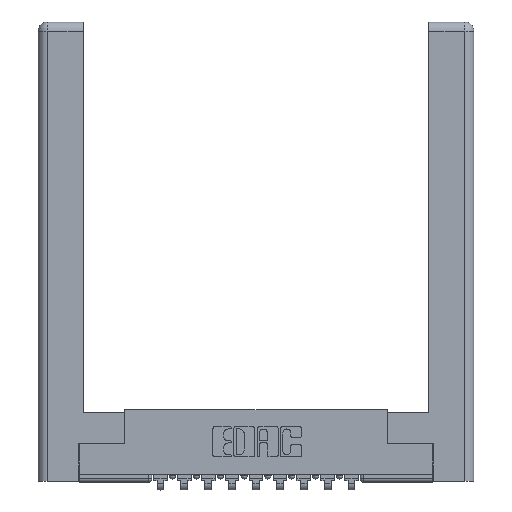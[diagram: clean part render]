
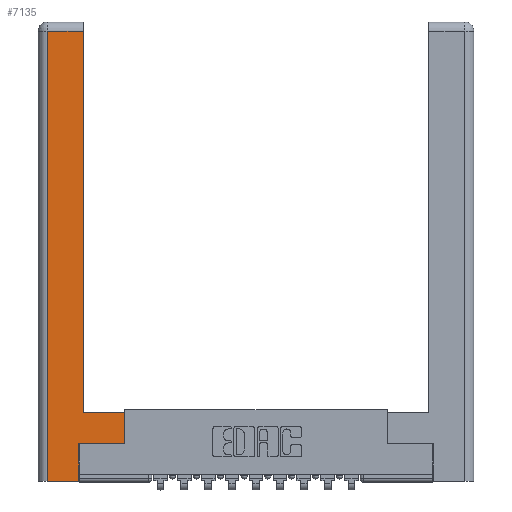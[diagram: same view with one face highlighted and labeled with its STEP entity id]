
A CAD part, top view. The second image highlights one B-rep face of the part: STEP entity #7135.
In plain terms, the highlighted planar face has unit normal (0, 0, 1).
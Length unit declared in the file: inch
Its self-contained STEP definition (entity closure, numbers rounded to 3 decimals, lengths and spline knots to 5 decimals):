
#481 = VECTOR ( 'NONE', #7855, 39.37008 ) ;
#577 = LINE ( 'NONE', #14822, #9826 ) ;
#635 = ORIENTED_EDGE ( 'NONE', *, *, #12212, .T. ) ;
#964 = VERTEX_POINT ( 'NONE', #5883 ) ;
#1213 = CARTESIAN_POINT ( 'NONE',  ( 0.0615, 2.94, 0. ) ) ;
#1228 = LINE ( 'NONE', #13345, #13043 ) ;
#1716 = FACE_OUTER_BOUND ( 'NONE', #7790, .T. ) ;
#1934 = ORIENTED_EDGE ( 'NONE', *, *, #13706, .T. ) ;
#2009 = CARTESIAN_POINT ( 'NONE',  ( 0.565, 0.245, 0. ) ) ;
#2551 = VERTEX_POINT ( 'NONE', #6103 ) ;
#3021 = PLANE ( 'NONE',  #4037 ) ;
#3238 = CARTESIAN_POINT ( 'NONE',  ( 0.565, 0.245, 0. ) ) ;
#3456 = ORIENTED_EDGE ( 'NONE', *, *, #12498, .T. ) ;
#4037 = AXIS2_PLACEMENT_3D ( 'NONE', #10258, #6478, #4224 ) ;
#4224 = DIRECTION ( 'NONE',  ( -1., 0., 0. ) ) ;
#4904 = CARTESIAN_POINT ( 'NONE',  ( 0.265, 0.245, 0. ) ) ;
#4952 = VECTOR ( 'NONE', #8055, 39.37008 ) ;
#5247 = EDGE_CURVE ( 'NONE', #8788, #11403, #8858, .T. ) ;
#5883 = CARTESIAN_POINT ( 'NONE',  ( 0.295, 0.45, 0. ) ) ;
#6103 = CARTESIAN_POINT ( 'NONE',  ( 0.265, 0., 0. ) ) ;
#6108 = ORIENTED_EDGE ( 'NONE', *, *, #14114, .T. ) ;
#6281 = DIRECTION ( 'NONE',  ( 1., 0., 0. ) ) ;
#6478 = DIRECTION ( 'NONE',  ( 0., 0., -1. ) ) ;
#6773 = LINE ( 'NONE', #9092, #481 ) ;
#6838 = ORIENTED_EDGE ( 'NONE', *, *, #13194, .T. ) ;
#6981 = LINE ( 'NONE', #10394, #9014 ) ;
#7135 = ADVANCED_FACE ( 'NONE', ( #1716 ), #3021, .F. ) ;
#7223 = DIRECTION ( 'NONE',  ( 0., 1., 0. ) ) ;
#7790 = EDGE_LOOP ( 'NONE', ( #6108, #635, #9020, #1934, #3456, #8652, #6838, #11118 ) ) ;
#7855 = DIRECTION ( 'NONE',  ( -1., 0., 0. ) ) ;
#8055 = DIRECTION ( 'NONE',  ( 1., 0., 0. ) ) ;
#8219 = LINE ( 'NONE', #13305, #9128 ) ;
#8366 = DIRECTION ( 'NONE',  ( 0., 1., 0. ) ) ;
#8652 = ORIENTED_EDGE ( 'NONE', *, *, #13442, .T. ) ;
#8788 = VERTEX_POINT ( 'NONE', #1213 ) ;
#8858 = LINE ( 'NONE', #14935, #10699 ) ;
#8957 = EDGE_CURVE ( 'NONE', #12801, #964, #577, .T. ) ;
#9014 = VECTOR ( 'NONE', #11666, 39.37008 ) ;
#9020 = ORIENTED_EDGE ( 'NONE', *, *, #5247, .T. ) ;
#9092 = CARTESIAN_POINT ( 'NONE',  ( 0.0615, 2.94, 0. ) ) ;
#9128 = VECTOR ( 'NONE', #8366, 39.37008 ) ;
#9530 = VECTOR ( 'NONE', #7223, 39.37008 ) ;
#9826 = VECTOR ( 'NONE', #12447, 39.37008 ) ;
#10258 = CARTESIAN_POINT ( 'NONE',  ( 0., 0., 0. ) ) ;
#10265 = DIRECTION ( 'NONE',  ( 0., -1., 0. ) ) ;
#10394 = CARTESIAN_POINT ( 'NONE',  ( 0.295, 3., 0. ) ) ;
#10699 = VECTOR ( 'NONE', #10265, 39.37008 ) ;
#10854 = LINE ( 'NONE', #3238, #4952 ) ;
#11009 = LINE ( 'NONE', #4904, #9530 ) ;
#11094 = VERTEX_POINT ( 'NONE', #12763 ) ;
#11118 = ORIENTED_EDGE ( 'NONE', *, *, #8957, .T. ) ;
#11166 = CARTESIAN_POINT ( 'NONE',  ( 0.0615, 0., 0. ) ) ;
#11403 = VERTEX_POINT ( 'NONE', #11166 ) ;
#11666 = DIRECTION ( 'NONE',  ( 0., 1., 0. ) ) ;
#12077 = VERTEX_POINT ( 'NONE', #14555 ) ;
#12212 = EDGE_CURVE ( 'NONE', #11094, #8788, #6773, .T. ) ;
#12447 = DIRECTION ( 'NONE',  ( -1., 0., 0. ) ) ;
#12498 = EDGE_CURVE ( 'NONE', #2551, #12077, #11009, .T. ) ;
#12722 = VERTEX_POINT ( 'NONE', #2009 ) ;
#12763 = CARTESIAN_POINT ( 'NONE',  ( 0.295, 2.94, 0. ) ) ;
#12801 = VERTEX_POINT ( 'NONE', #13625 ) ;
#13043 = VECTOR ( 'NONE', #6281, 39.37008 ) ;
#13194 = EDGE_CURVE ( 'NONE', #12722, #12801, #8219, .T. ) ;
#13305 = CARTESIAN_POINT ( 'NONE',  ( 0.565, 0.45, 0. ) ) ;
#13345 = CARTESIAN_POINT ( 'NONE',  ( 0.265, 0., 0. ) ) ;
#13442 = EDGE_CURVE ( 'NONE', #12077, #12722, #10854, .T. ) ;
#13625 = CARTESIAN_POINT ( 'NONE',  ( 0.565, 0.45, 0. ) ) ;
#13706 = EDGE_CURVE ( 'NONE', #11403, #2551, #1228, .T. ) ;
#14114 = EDGE_CURVE ( 'NONE', #964, #11094, #6981, .T. ) ;
#14555 = CARTESIAN_POINT ( 'NONE',  ( 0.265, 0.245, 0. ) ) ;
#14822 = CARTESIAN_POINT ( 'NONE',  ( 0.295, 0.45, 0. ) ) ;
#14935 = CARTESIAN_POINT ( 'NONE',  ( 0.0615, 0., 0. ) ) ;
